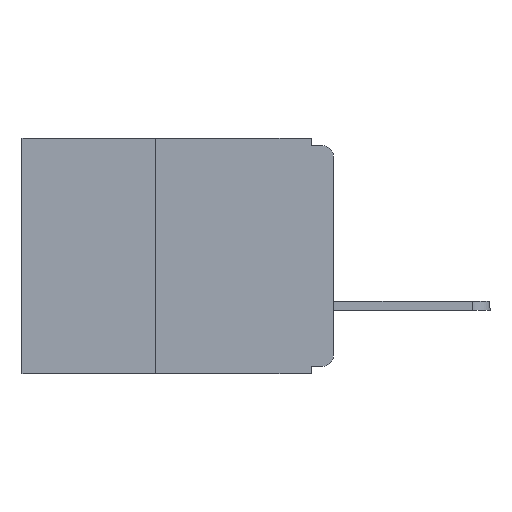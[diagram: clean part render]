
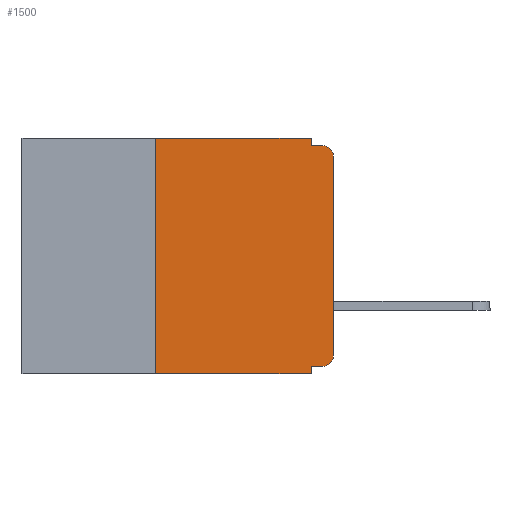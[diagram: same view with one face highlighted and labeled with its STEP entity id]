
A CAD part, left-side view. The second image highlights one B-rep face of the part: STEP entity #1500.
In plain terms, the highlighted planar face has unit normal (-1, 0, 0).
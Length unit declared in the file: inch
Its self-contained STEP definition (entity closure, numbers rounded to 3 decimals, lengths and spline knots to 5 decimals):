
#382 = DIRECTION ( 'NONE',  ( 0., 0., -1. ) ) ;
#1176 = DIRECTION ( 'NONE',  ( 0., 0., 1. ) ) ;
#1414 = AXIS2_PLACEMENT_3D ( 'NONE', #31242, #15627, #33832 ) ;
#1500 = ADVANCED_FACE ( 'NONE', ( #26941 ), #12107, .F. ) ;
#1797 = AXIS2_PLACEMENT_3D ( 'NONE', #21368, #12104, #5116 ) ;
#2023 = VERTEX_POINT ( 'NONE', #26891 ) ;
#2084 = EDGE_CURVE ( 'NONE', #3593, #3288, #22798, .T. ) ;
#2921 = VERTEX_POINT ( 'NONE', #14855 ) ;
#3190 = ORIENTED_EDGE ( 'NONE', *, *, #24745, .T. ) ;
#3288 = VERTEX_POINT ( 'NONE', #32470 ) ;
#3332 = VERTEX_POINT ( 'NONE', #32101 ) ;
#3593 = VERTEX_POINT ( 'NONE', #26715 ) ;
#4502 = VERTEX_POINT ( 'NONE', #11335 ) ;
#5116 = DIRECTION ( 'NONE',  ( 0., 0., -1. ) ) ;
#5172 = AXIS2_PLACEMENT_3D ( 'NONE', #13422, #31684, #16069 ) ;
#6429 = ORIENTED_EDGE ( 'NONE', *, *, #15192, .T. ) ;
#6746 = VECTOR ( 'NONE', #17313, 39.37008 ) ;
#6776 = LINE ( 'NONE', #26591, #33850 ) ;
#7261 = CARTESIAN_POINT ( 'NONE',  ( 0., 0.25, -0.33 ) ) ;
#7337 = VERTEX_POINT ( 'NONE', #15704 ) ;
#8769 = VECTOR ( 'NONE', #26052, 39.37008 ) ;
#8805 = EDGE_CURVE ( 'NONE', #4502, #2023, #22465, .T. ) ;
#8830 = CARTESIAN_POINT ( 'NONE',  ( 0., 0.015, -0.32 ) ) ;
#9250 = LINE ( 'NONE', #24761, #22453 ) ;
#10690 = DIRECTION ( 'NONE',  ( 0., -1., 0. ) ) ;
#11335 = CARTESIAN_POINT ( 'NONE',  ( 0., 0.031, -0.01 ) ) ;
#12046 = ORIENTED_EDGE ( 'NONE', *, *, #33583, .T. ) ;
#12104 = DIRECTION ( 'NONE',  ( 1., 0., 0. ) ) ;
#12107 = PLANE ( 'NONE',  #1797 ) ;
#13188 = CIRCLE ( 'NONE', #5172, 0.015 ) ;
#13422 = CARTESIAN_POINT ( 'NONE',  ( 0., 0.015, -0.025 ) ) ;
#14589 = ORIENTED_EDGE ( 'NONE', *, *, #21170, .F. ) ;
#14675 = CARTESIAN_POINT ( 'NONE',  ( 0., 0.25, -0.33 ) ) ;
#14855 = CARTESIAN_POINT ( 'NONE',  ( 0., 0., -0.305 ) ) ;
#15192 = EDGE_CURVE ( 'NONE', #2921, #32024, #9250, .T. ) ;
#15278 = EDGE_CURVE ( 'NONE', #27437, #3332, #26957, .T. ) ;
#15423 = ORIENTED_EDGE ( 'NONE', *, *, #2084, .F. ) ;
#15448 = DIRECTION ( 'NONE',  ( 0., -1., 0. ) ) ;
#15506 = VECTOR ( 'NONE', #21049, 39.37008 ) ;
#15524 = VECTOR ( 'NONE', #33465, 39.37008 ) ;
#15627 = DIRECTION ( 'NONE',  ( -1., 0., 0. ) ) ;
#15704 = CARTESIAN_POINT ( 'NONE',  ( 0., 0.031, 0. ) ) ;
#16069 = DIRECTION ( 'NONE',  ( 0., 0., -1. ) ) ;
#17130 = ORIENTED_EDGE ( 'NONE', *, *, #8805, .F. ) ;
#17313 = DIRECTION ( 'NONE',  ( 0., 0., 1. ) ) ;
#17661 = ORIENTED_EDGE ( 'NONE', *, *, #25083, .F. ) ;
#18083 = CARTESIAN_POINT ( 'NONE',  ( 0., 0.031, -0.33 ) ) ;
#18391 = EDGE_CURVE ( 'NONE', #32024, #2023, #13188, .T. ) ;
#18412 = CARTESIAN_POINT ( 'NONE',  ( 0., 0., -0.01 ) ) ;
#18559 = CARTESIAN_POINT ( 'NONE',  ( 0., 0.437, -0.33 ) ) ;
#18854 = VECTOR ( 'NONE', #15448, 39.37008 ) ;
#19683 = LINE ( 'NONE', #28461, #18854 ) ;
#20623 = EDGE_LOOP ( 'NONE', ( #6429, #30512, #17130, #30125, #17661, #25176, #12046, #15423, #14589, #3190 ) ) ;
#21049 = DIRECTION ( 'NONE',  ( 0., -1., 0. ) ) ;
#21170 = EDGE_CURVE ( 'NONE', #33774, #3593, #30216, .T. ) ;
#21368 = CARTESIAN_POINT ( 'NONE',  ( 0., 0.437, 0. ) ) ;
#22270 = LINE ( 'NONE', #18559, #29182 ) ;
#22453 = VECTOR ( 'NONE', #1176, 39.37008 ) ;
#22465 = LINE ( 'NONE', #18412, #15506 ) ;
#22570 = CIRCLE ( 'NONE', #1414, 0.015 ) ;
#22798 = LINE ( 'NONE', #18083, #8769 ) ;
#24745 = EDGE_CURVE ( 'NONE', #33774, #2921, #22570, .T. ) ;
#24761 = CARTESIAN_POINT ( 'NONE',  ( 0., 0., 0. ) ) ;
#25083 = EDGE_CURVE ( 'NONE', #3332, #7337, #19683, .T. ) ;
#25176 = ORIENTED_EDGE ( 'NONE', *, *, #15278, .F. ) ;
#26052 = DIRECTION ( 'NONE',  ( 0., 0., -1. ) ) ;
#26591 = CARTESIAN_POINT ( 'NONE',  ( 0., 0.031, 0. ) ) ;
#26715 = CARTESIAN_POINT ( 'NONE',  ( 0., 0.031, -0.32 ) ) ;
#26891 = CARTESIAN_POINT ( 'NONE',  ( 0., 0.015, -0.01 ) ) ;
#26941 = FACE_OUTER_BOUND ( 'NONE', #20623, .T. ) ;
#26957 = LINE ( 'NONE', #14675, #6746 ) ;
#27437 = VERTEX_POINT ( 'NONE', #7261 ) ;
#27680 = CARTESIAN_POINT ( 'NONE',  ( 0., 0., -0.025 ) ) ;
#28263 = CARTESIAN_POINT ( 'NONE',  ( 0., 0., -0.32 ) ) ;
#28461 = CARTESIAN_POINT ( 'NONE',  ( 0., 0.437, 0. ) ) ;
#29182 = VECTOR ( 'NONE', #10690, 39.37008 ) ;
#29993 = EDGE_CURVE ( 'NONE', #7337, #4502, #6776, .T. ) ;
#30125 = ORIENTED_EDGE ( 'NONE', *, *, #29993, .F. ) ;
#30216 = LINE ( 'NONE', #28263, #15524 ) ;
#30512 = ORIENTED_EDGE ( 'NONE', *, *, #18391, .T. ) ;
#31242 = CARTESIAN_POINT ( 'NONE',  ( 0., 0.015, -0.305 ) ) ;
#31684 = DIRECTION ( 'NONE',  ( -1., 0., 0. ) ) ;
#32024 = VERTEX_POINT ( 'NONE', #27680 ) ;
#32101 = CARTESIAN_POINT ( 'NONE',  ( 0., 0.25, 0. ) ) ;
#32470 = CARTESIAN_POINT ( 'NONE',  ( 0., 0.031, -0.33 ) ) ;
#33465 = DIRECTION ( 'NONE',  ( 0., 1., 0. ) ) ;
#33583 = EDGE_CURVE ( 'NONE', #27437, #3288, #22270, .T. ) ;
#33774 = VERTEX_POINT ( 'NONE', #8830 ) ;
#33832 = DIRECTION ( 'NONE',  ( 0., 0., -1. ) ) ;
#33850 = VECTOR ( 'NONE', #382, 39.37008 ) ;
